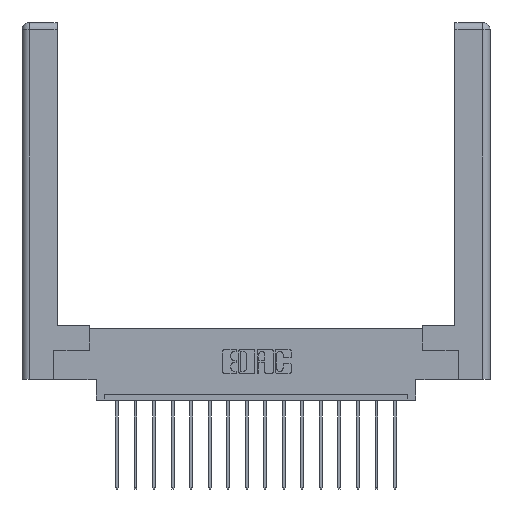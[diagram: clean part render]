
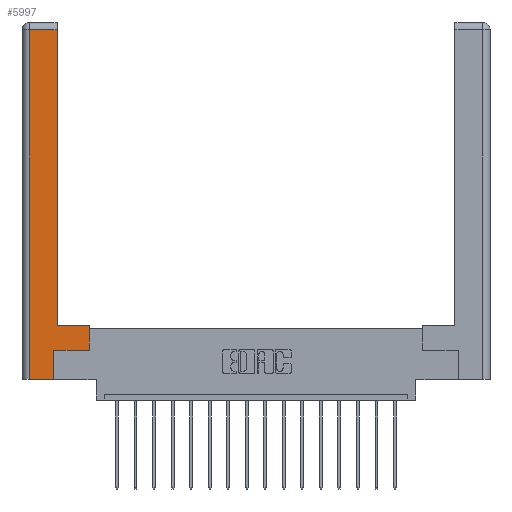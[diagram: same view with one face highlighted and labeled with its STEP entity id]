
A CAD part, top view. The second image highlights one B-rep face of the part: STEP entity #5997.
In plain terms, the highlighted planar face has unit normal (0, 0, 1).
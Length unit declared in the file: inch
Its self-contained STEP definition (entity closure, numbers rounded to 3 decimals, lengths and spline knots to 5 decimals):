
#378 = CARTESIAN_POINT ( 'NONE',  ( 0.565, 0.245, 0. ) ) ;
#689 = CARTESIAN_POINT ( 'NONE',  ( 0.295, 0.45, 0. ) ) ;
#719 = VECTOR ( 'NONE', #10105, 39.37008 ) ;
#735 = ORIENTED_EDGE ( 'NONE', *, *, #10109, .T. ) ;
#760 = VERTEX_POINT ( 'NONE', #10874 ) ;
#1160 = CARTESIAN_POINT ( 'NONE',  ( 0.265, 0., 0. ) ) ;
#1194 = VERTEX_POINT ( 'NONE', #2077 ) ;
#1238 = ORIENTED_EDGE ( 'NONE', *, *, #10973, .T. ) ;
#1418 = EDGE_CURVE ( 'NONE', #2118, #6695, #9307, .T. ) ;
#1517 = ORIENTED_EDGE ( 'NONE', *, *, #1418, .T. ) ;
#2016 = ORIENTED_EDGE ( 'NONE', *, *, #9120, .T. ) ;
#2077 = CARTESIAN_POINT ( 'NONE',  ( 0.265, 0.245, 0. ) ) ;
#2118 = VERTEX_POINT ( 'NONE', #2306 ) ;
#2306 = CARTESIAN_POINT ( 'NONE',  ( 0.0615, 0., 0. ) ) ;
#2524 = CARTESIAN_POINT ( 'NONE',  ( 0.0615, 2.94, 0. ) ) ;
#2693 = DIRECTION ( 'NONE',  ( -1., 0., 0. ) ) ;
#2781 = CARTESIAN_POINT ( 'NONE',  ( 0.0615, 0., 0. ) ) ;
#3395 = CARTESIAN_POINT ( 'NONE',  ( 0.0615, 2.94, 0. ) ) ;
#4067 = DIRECTION ( 'NONE',  ( 1., 0., 0. ) ) ;
#5019 = EDGE_CURVE ( 'NONE', #1194, #8563, #7017, .T. ) ;
#5168 = VECTOR ( 'NONE', #8741, 39.37008 ) ;
#5588 = VECTOR ( 'NONE', #4067, 39.37008 ) ;
#5816 = LINE ( 'NONE', #12886, #5168 ) ;
#5945 = LINE ( 'NONE', #2781, #12918 ) ;
#5997 = ADVANCED_FACE ( 'NONE', ( #14838 ), #7996, .F. ) ;
#6430 = VECTOR ( 'NONE', #8971, 39.37008 ) ;
#6663 = LINE ( 'NONE', #13575, #16892 ) ;
#6695 = VERTEX_POINT ( 'NONE', #1160 ) ;
#7017 = LINE ( 'NONE', #378, #719 ) ;
#7377 = LINE ( 'NONE', #11275, #14366 ) ;
#7788 = CARTESIAN_POINT ( 'NONE',  ( 0.565, 0.245, 0. ) ) ;
#7996 = PLANE ( 'NONE',  #16483 ) ;
#8563 = VERTEX_POINT ( 'NONE', #7788 ) ;
#8741 = DIRECTION ( 'NONE',  ( 0., 1., 0. ) ) ;
#8971 = DIRECTION ( 'NONE',  ( 0., 1., 0. ) ) ;
#9061 = DIRECTION ( 'NONE',  ( -1., 0., 0. ) ) ;
#9120 = EDGE_CURVE ( 'NONE', #760, #14654, #7377, .T. ) ;
#9307 = LINE ( 'NONE', #16668, #5588 ) ;
#9461 = DIRECTION ( 'NONE',  ( -1., 0., 0. ) ) ;
#9729 = LINE ( 'NONE', #3395, #14742 ) ;
#10105 = DIRECTION ( 'NONE',  ( 1., 0., 0. ) ) ;
#10109 = EDGE_CURVE ( 'NONE', #8563, #760, #5816, .T. ) ;
#10569 = LINE ( 'NONE', #13046, #6430 ) ;
#10706 = DIRECTION ( 'NONE',  ( 0., 1., 0. ) ) ;
#10716 = DIRECTION ( 'NONE',  ( 0., -1., 0. ) ) ;
#10874 = CARTESIAN_POINT ( 'NONE',  ( 0.565, 0.45, 0. ) ) ;
#10966 = CARTESIAN_POINT ( 'NONE',  ( 0., 0., 0. ) ) ;
#10973 = EDGE_CURVE ( 'NONE', #6695, #1194, #6663, .T. ) ;
#11275 = CARTESIAN_POINT ( 'NONE',  ( 0.295, 0.45, 0. ) ) ;
#11843 = ORIENTED_EDGE ( 'NONE', *, *, #15865, .T. ) ;
#12108 = VERTEX_POINT ( 'NONE', #14942 ) ;
#12886 = CARTESIAN_POINT ( 'NONE',  ( 0.565, 0.45, 0. ) ) ;
#12918 = VECTOR ( 'NONE', #10716, 39.37008 ) ;
#13046 = CARTESIAN_POINT ( 'NONE',  ( 0.295, 3., 0. ) ) ;
#13575 = CARTESIAN_POINT ( 'NONE',  ( 0.265, 0.245, 0. ) ) ;
#14366 = VECTOR ( 'NONE', #2693, 39.37008 ) ;
#14654 = VERTEX_POINT ( 'NONE', #689 ) ;
#14742 = VECTOR ( 'NONE', #9061, 39.37008 ) ;
#14838 = FACE_OUTER_BOUND ( 'NONE', #16636, .T. ) ;
#14942 = CARTESIAN_POINT ( 'NONE',  ( 0.295, 2.94, 0. ) ) ;
#15056 = DIRECTION ( 'NONE',  ( 0., 0., -1. ) ) ;
#15398 = EDGE_CURVE ( 'NONE', #12108, #17595, #9729, .T. ) ;
#15865 = EDGE_CURVE ( 'NONE', #14654, #12108, #10569, .T. ) ;
#16279 = ORIENTED_EDGE ( 'NONE', *, *, #5019, .T. ) ;
#16483 = AXIS2_PLACEMENT_3D ( 'NONE', #10966, #15056, #9461 ) ;
#16571 = ORIENTED_EDGE ( 'NONE', *, *, #15398, .T. ) ;
#16636 = EDGE_LOOP ( 'NONE', ( #11843, #16571, #17940, #1517, #1238, #16279, #735, #2016 ) ) ;
#16668 = CARTESIAN_POINT ( 'NONE',  ( 0.265, 0., 0. ) ) ;
#16892 = VECTOR ( 'NONE', #10706, 39.37008 ) ;
#17125 = EDGE_CURVE ( 'NONE', #17595, #2118, #5945, .T. ) ;
#17595 = VERTEX_POINT ( 'NONE', #2524 ) ;
#17940 = ORIENTED_EDGE ( 'NONE', *, *, #17125, .T. ) ;
